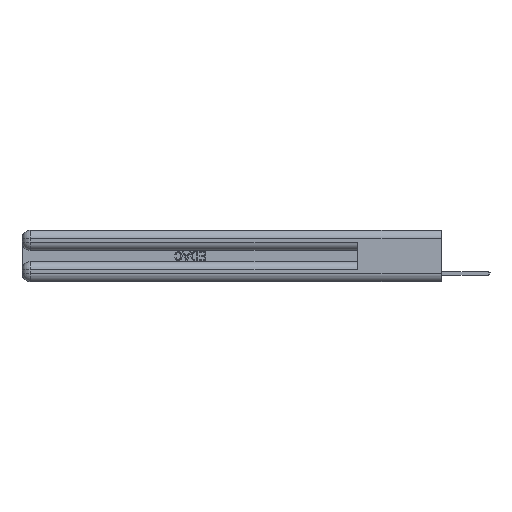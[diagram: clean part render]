
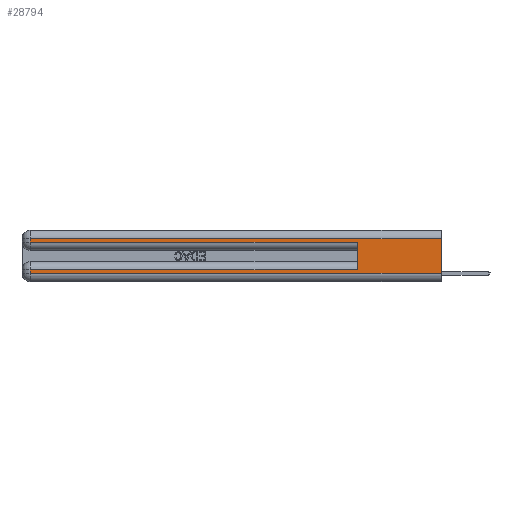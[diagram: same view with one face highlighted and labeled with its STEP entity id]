
A CAD part, left-side view. The second image highlights one B-rep face of the part: STEP entity #28794.
In plain terms, the highlighted planar face has unit normal (-1, 0, 0).
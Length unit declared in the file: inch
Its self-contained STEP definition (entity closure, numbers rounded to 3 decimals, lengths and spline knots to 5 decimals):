
#253 = LINE ( 'NONE', #5733, #20834 ) ;
#786 = EDGE_CURVE ( 'NONE', #7824, #10504, #2192, .T. ) ;
#1923 = LINE ( 'NONE', #5995, #33780 ) ;
#2192 = LINE ( 'NONE', #30354, #26980 ) ;
#2443 = DIRECTION ( 'NONE',  ( 0., 0., -1. ) ) ;
#2451 = EDGE_CURVE ( 'NONE', #10600, #7376, #11277, .T. ) ;
#2493 = CARTESIAN_POINT ( 'NONE',  ( 0., 0., 0.37 ) ) ;
#3434 = CARTESIAN_POINT ( 'NONE',  ( 0., 0., 0.06 ) ) ;
#4082 = VECTOR ( 'NONE', #5628, 39.37008 ) ;
#5276 = DIRECTION ( 'NONE',  ( 0., 1., 0. ) ) ;
#5398 = FACE_OUTER_BOUND ( 'NONE', #6793, .T. ) ;
#5628 = DIRECTION ( 'NONE',  ( 0., 1., 0. ) ) ;
#5733 = CARTESIAN_POINT ( 'NONE',  ( 0., 0., 0.31 ) ) ;
#5995 = CARTESIAN_POINT ( 'NONE',  ( 0., 0.6, 0.145 ) ) ;
#6793 = EDGE_LOOP ( 'NONE', ( #22266, #18166, #22005, #10137, #29503, #31142, #11139, #16224 ) ) ;
#7376 = VERTEX_POINT ( 'NONE', #21568 ) ;
#7824 = VERTEX_POINT ( 'NONE', #34688 ) ;
#8132 = EDGE_CURVE ( 'NONE', #31036, #29308, #21031, .T. ) ;
#8971 = EDGE_CURVE ( 'NONE', #7376, #31036, #18872, .T. ) ;
#9426 = CARTESIAN_POINT ( 'NONE',  ( 0., 0.6, 0.085 ) ) ;
#10137 = ORIENTED_EDGE ( 'NONE', *, *, #786, .T. ) ;
#10460 = LINE ( 'NONE', #12835, #30942 ) ;
#10504 = VERTEX_POINT ( 'NONE', #34581 ) ;
#10600 = VERTEX_POINT ( 'NONE', #9426 ) ;
#11139 = ORIENTED_EDGE ( 'NONE', *, *, #8971, .T. ) ;
#11207 = EDGE_CURVE ( 'NONE', #15065, #21792, #253, .T. ) ;
#11277 = LINE ( 'NONE', #27207, #4082 ) ;
#11571 = DIRECTION ( 'NONE',  ( 0., -1., 0. ) ) ;
#12448 = CARTESIAN_POINT ( 'NONE',  ( 0., 2.94, 0.31 ) ) ;
#12569 = VECTOR ( 'NONE', #2443, 39.37008 ) ;
#12784 = CARTESIAN_POINT ( 'NONE',  ( 0., 2.94, 0.06 ) ) ;
#12835 = CARTESIAN_POINT ( 'NONE',  ( 0., 2.94, 0.37 ) ) ;
#13883 = VECTOR ( 'NONE', #11571, 39.37008 ) ;
#14638 = CARTESIAN_POINT ( 'NONE',  ( 0., 0., 0.06 ) ) ;
#15065 = VERTEX_POINT ( 'NONE', #16324 ) ;
#15327 = VECTOR ( 'NONE', #16703, 39.37008 ) ;
#16014 = DIRECTION ( 'NONE',  ( 1., 0., 0. ) ) ;
#16224 = ORIENTED_EDGE ( 'NONE', *, *, #8132, .T. ) ;
#16324 = CARTESIAN_POINT ( 'NONE',  ( 0., 0., 0.31 ) ) ;
#16587 = CARTESIAN_POINT ( 'NONE',  ( 0., 0., 0.37 ) ) ;
#16703 = DIRECTION ( 'NONE',  ( 0., 0., -1. ) ) ;
#18166 = ORIENTED_EDGE ( 'NONE', *, *, #11207, .T. ) ;
#18872 = LINE ( 'NONE', #29626, #12569 ) ;
#19956 = LINE ( 'NONE', #16587, #15327 ) ;
#20834 = VECTOR ( 'NONE', #5276, 39.37008 ) ;
#21031 = LINE ( 'NONE', #3434, #13883 ) ;
#21568 = CARTESIAN_POINT ( 'NONE',  ( 0., 2.94, 0.085 ) ) ;
#21792 = VERTEX_POINT ( 'NONE', #12448 ) ;
#21849 = DIRECTION ( 'NONE',  ( 0., -1., 0. ) ) ;
#21944 = DIRECTION ( 'NONE',  ( 0., 0., -1. ) ) ;
#22005 = ORIENTED_EDGE ( 'NONE', *, *, #26717, .T. ) ;
#22266 = ORIENTED_EDGE ( 'NONE', *, *, #31982, .F. ) ;
#24757 = DIRECTION ( 'NONE',  ( 0., 0., 1. ) ) ;
#26717 = EDGE_CURVE ( 'NONE', #21792, #7824, #10460, .T. ) ;
#26980 = VECTOR ( 'NONE', #21849, 39.37008 ) ;
#27207 = CARTESIAN_POINT ( 'NONE',  ( 0., 0., 0.085 ) ) ;
#28794 = ADVANCED_FACE ( 'NONE', ( #5398 ), #31903, .F. ) ;
#29308 = VERTEX_POINT ( 'NONE', #14638 ) ;
#29503 = ORIENTED_EDGE ( 'NONE', *, *, #30212, .F. ) ;
#29626 = CARTESIAN_POINT ( 'NONE',  ( 0., 2.94, 0.37 ) ) ;
#29912 = AXIS2_PLACEMENT_3D ( 'NONE', #2493, #16014, #21944 ) ;
#30212 = EDGE_CURVE ( 'NONE', #10600, #10504, #1923, .T. ) ;
#30354 = CARTESIAN_POINT ( 'NONE',  ( 0., 0., 0.285 ) ) ;
#30942 = VECTOR ( 'NONE', #31651, 39.37008 ) ;
#31036 = VERTEX_POINT ( 'NONE', #12784 ) ;
#31142 = ORIENTED_EDGE ( 'NONE', *, *, #2451, .T. ) ;
#31651 = DIRECTION ( 'NONE',  ( 0., 0., -1. ) ) ;
#31903 = PLANE ( 'NONE',  #29912 ) ;
#31982 = EDGE_CURVE ( 'NONE', #15065, #29308, #19956, .T. ) ;
#33780 = VECTOR ( 'NONE', #24757, 39.37008 ) ;
#34581 = CARTESIAN_POINT ( 'NONE',  ( 0., 0.6, 0.285 ) ) ;
#34688 = CARTESIAN_POINT ( 'NONE',  ( 0., 2.94, 0.285 ) ) ;
